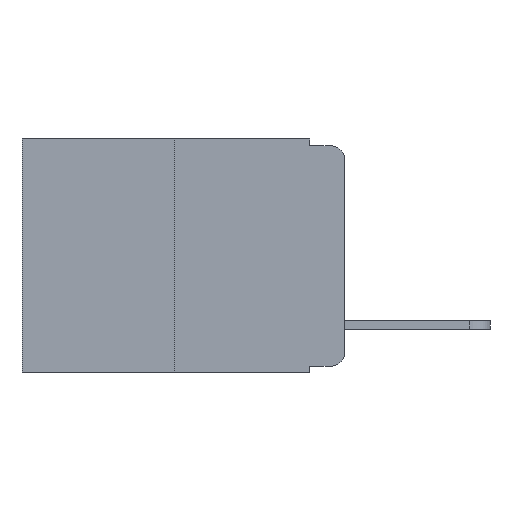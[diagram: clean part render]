
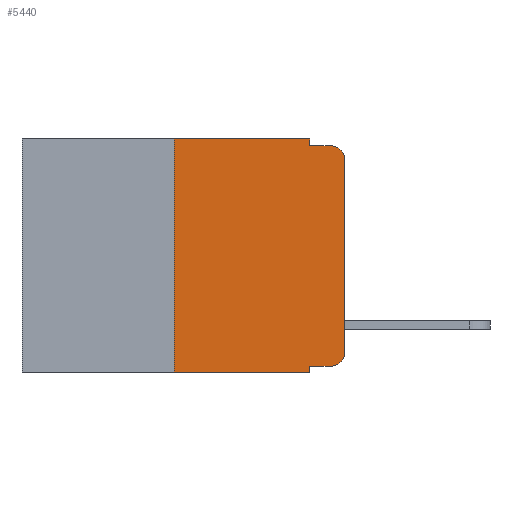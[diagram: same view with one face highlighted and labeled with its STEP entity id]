
A CAD part, left-side view. The second image highlights one B-rep face of the part: STEP entity #5440.
In plain terms, the highlighted planar face has unit normal (-1, 0, 0).
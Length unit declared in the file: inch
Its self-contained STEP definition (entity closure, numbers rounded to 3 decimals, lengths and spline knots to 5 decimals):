
#103 = VECTOR ( 'NONE', #6795, 39.37008 ) ;
#306 = CIRCLE ( 'NONE', #6207, 0.02 ) ;
#488 = CARTESIAN_POINT ( 'NONE',  ( 0., 0.051, 0. ) ) ;
#497 = LINE ( 'NONE', #488, #103 ) ;
#764 = EDGE_CURVE ( 'NONE', #2041, #9177, #8443, .T. ) ;
#1091 = ORIENTED_EDGE ( 'NONE', *, *, #4583, .T. ) ;
#1207 = LINE ( 'NONE', #3158, #14506 ) ;
#1282 = CARTESIAN_POINT ( 'NONE',  ( 0., 0.02, -0.313 ) ) ;
#1444 = AXIS2_PLACEMENT_3D ( 'NONE', #1282, #10305, #2579 ) ;
#1508 = CARTESIAN_POINT ( 'NONE',  ( 0., 0.02, -0.03 ) ) ;
#1528 = CARTESIAN_POINT ( 'NONE',  ( 0., 0.051, -0.343 ) ) ;
#1683 = CARTESIAN_POINT ( 'NONE',  ( 0., 0.473, 0. ) ) ;
#1836 = EDGE_CURVE ( 'NONE', #16615, #14608, #7450, .T. ) ;
#2027 = ORIENTED_EDGE ( 'NONE', *, *, #3801, .F. ) ;
#2041 = VERTEX_POINT ( 'NONE', #12543 ) ;
#2336 = CARTESIAN_POINT ( 'NONE',  ( 0., 0.051, -0.01 ) ) ;
#2579 = DIRECTION ( 'NONE',  ( 0., 0., -1. ) ) ;
#2639 = ORIENTED_EDGE ( 'NONE', *, *, #764, .T. ) ;
#2750 = DIRECTION ( 'NONE',  ( 0., -1., 0. ) ) ;
#2987 = VECTOR ( 'NONE', #2750, 39.37008 ) ;
#3119 = VECTOR ( 'NONE', #12656, 39.37008 ) ;
#3158 = CARTESIAN_POINT ( 'NONE',  ( 0., 0.473, -0.343 ) ) ;
#3570 = EDGE_CURVE ( 'NONE', #7351, #10906, #497, .T. ) ;
#3801 = EDGE_CURVE ( 'NONE', #7073, #8552, #6741, .T. ) ;
#3810 = VECTOR ( 'NONE', #15795, 39.37008 ) ;
#3829 = ORIENTED_EDGE ( 'NONE', *, *, #5399, .T. ) ;
#3968 = VECTOR ( 'NONE', #6790, 39.37008 ) ;
#4583 = EDGE_CURVE ( 'NONE', #7351, #4974, #13854, .T. ) ;
#4699 = CARTESIAN_POINT ( 'NONE',  ( 0., 0.25, 0. ) ) ;
#4963 = EDGE_LOOP ( 'NONE', ( #2639, #3829, #13725, #7832, #7288, #2027, #12921, #10558, #1091, #15049 ) ) ;
#4974 = VERTEX_POINT ( 'NONE', #10778 ) ;
#5399 = EDGE_CURVE ( 'NONE', #9177, #8777, #306, .T. ) ;
#5436 = DIRECTION ( 'NONE',  ( 0., 0., -1. ) ) ;
#5440 = ADVANCED_FACE ( 'NONE', ( #15023 ), #8213, .F. ) ;
#5727 = CARTESIAN_POINT ( 'NONE',  ( 0., 0.473, 0. ) ) ;
#6207 = AXIS2_PLACEMENT_3D ( 'NONE', #1508, #14410, #5436 ) ;
#6268 = CARTESIAN_POINT ( 'NONE',  ( 0., 0.051, 0. ) ) ;
#6431 = LINE ( 'NONE', #1683, #2987 ) ;
#6741 = LINE ( 'NONE', #4699, #3119 ) ;
#6790 = DIRECTION ( 'NONE',  ( 0., 0., -1. ) ) ;
#6795 = DIRECTION ( 'NONE',  ( 0., 0., -1. ) ) ;
#6944 = CARTESIAN_POINT ( 'NONE',  ( 0., 0.02, -0.01 ) ) ;
#7073 = VERTEX_POINT ( 'NONE', #11261 ) ;
#7158 = DIRECTION ( 'NONE',  ( 0., 0., -1. ) ) ;
#7288 = ORIENTED_EDGE ( 'NONE', *, *, #9763, .F. ) ;
#7351 = VERTEX_POINT ( 'NONE', #9380 ) ;
#7414 = DIRECTION ( 'NONE',  ( 0., 0., 1. ) ) ;
#7450 = LINE ( 'NONE', #9537, #3968 ) ;
#7832 = ORIENTED_EDGE ( 'NONE', *, *, #1836, .F. ) ;
#8213 = PLANE ( 'NONE',  #11391 ) ;
#8443 = LINE ( 'NONE', #16202, #11259 ) ;
#8552 = VERTEX_POINT ( 'NONE', #14428 ) ;
#8777 = VERTEX_POINT ( 'NONE', #6944 ) ;
#8828 = DIRECTION ( 'NONE',  ( 0., -1., 0. ) ) ;
#8900 = LINE ( 'NONE', #13426, #3810 ) ;
#9177 = VERTEX_POINT ( 'NONE', #13059 ) ;
#9380 = CARTESIAN_POINT ( 'NONE',  ( 0., 0.051, -0.333 ) ) ;
#9537 = CARTESIAN_POINT ( 'NONE',  ( 0., 0.051, 0. ) ) ;
#9763 = EDGE_CURVE ( 'NONE', #8552, #16615, #6431, .T. ) ;
#10305 = DIRECTION ( 'NONE',  ( -1., 0., 0. ) ) ;
#10558 = ORIENTED_EDGE ( 'NONE', *, *, #3570, .F. ) ;
#10778 = CARTESIAN_POINT ( 'NONE',  ( 0., 0.02, -0.333 ) ) ;
#10794 = CIRCLE ( 'NONE', #1444, 0.02 ) ;
#10906 = VERTEX_POINT ( 'NONE', #1528 ) ;
#10964 = EDGE_CURVE ( 'NONE', #14608, #8777, #8900, .T. ) ;
#11072 = EDGE_CURVE ( 'NONE', #7073, #10906, #1207, .T. ) ;
#11259 = VECTOR ( 'NONE', #7414, 39.37008 ) ;
#11261 = CARTESIAN_POINT ( 'NONE',  ( 0., 0.25, -0.343 ) ) ;
#11391 = AXIS2_PLACEMENT_3D ( 'NONE', #5727, #14804, #7158 ) ;
#12543 = CARTESIAN_POINT ( 'NONE',  ( 0., 0., -0.313 ) ) ;
#12656 = DIRECTION ( 'NONE',  ( 0., 0., 1. ) ) ;
#12921 = ORIENTED_EDGE ( 'NONE', *, *, #11072, .T. ) ;
#13059 = CARTESIAN_POINT ( 'NONE',  ( 0., 0., -0.03 ) ) ;
#13426 = CARTESIAN_POINT ( 'NONE',  ( 0., 0.051, -0.01 ) ) ;
#13440 = VECTOR ( 'NONE', #8828, 39.37008 ) ;
#13725 = ORIENTED_EDGE ( 'NONE', *, *, #10964, .F. ) ;
#13854 = LINE ( 'NONE', #16422, #13440 ) ;
#14090 = EDGE_CURVE ( 'NONE', #4974, #2041, #10794, .T. ) ;
#14410 = DIRECTION ( 'NONE',  ( -1., 0., 0. ) ) ;
#14428 = CARTESIAN_POINT ( 'NONE',  ( 0., 0.25, 0. ) ) ;
#14506 = VECTOR ( 'NONE', #16251, 39.37008 ) ;
#14608 = VERTEX_POINT ( 'NONE', #2336 ) ;
#14804 = DIRECTION ( 'NONE',  ( 1., 0., 0. ) ) ;
#15023 = FACE_OUTER_BOUND ( 'NONE', #4963, .T. ) ;
#15049 = ORIENTED_EDGE ( 'NONE', *, *, #14090, .T. ) ;
#15795 = DIRECTION ( 'NONE',  ( 0., -1., 0. ) ) ;
#16202 = CARTESIAN_POINT ( 'NONE',  ( 0., 0., 0. ) ) ;
#16251 = DIRECTION ( 'NONE',  ( 0., -1., 0. ) ) ;
#16422 = CARTESIAN_POINT ( 'NONE',  ( 0., 0.051, -0.333 ) ) ;
#16615 = VERTEX_POINT ( 'NONE', #6268 ) ;
